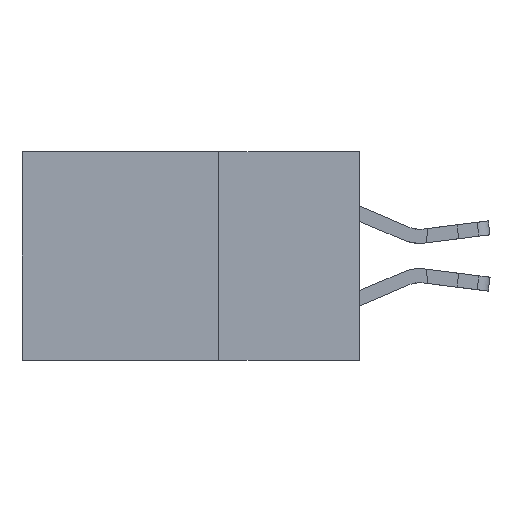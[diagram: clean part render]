
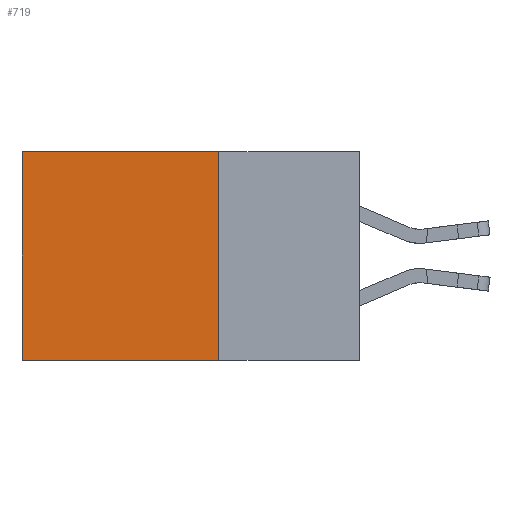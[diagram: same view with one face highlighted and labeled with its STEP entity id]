
A CAD part, left-side view. The second image highlights one B-rep face of the part: STEP entity #719.
In plain terms, the highlighted planar face has unit normal (-1, 0, 0).
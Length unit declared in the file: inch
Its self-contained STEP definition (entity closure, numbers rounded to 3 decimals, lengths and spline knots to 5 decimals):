
#719 = ADVANCED_FACE ( 'NONE', ( #21245 ), #32549, .F. ) ;
#754 = EDGE_CURVE ( 'NONE', #16952, #25200, #29790, .T. ) ;
#1808 = CARTESIAN_POINT ( 'NONE',  ( 0.2875, 0.25, 0. ) ) ;
#2608 = ORIENTED_EDGE ( 'NONE', *, *, #5707, .F. ) ;
#3145 = EDGE_CURVE ( 'NONE', #32842, #32727, #15800, .T. ) ;
#4558 = CARTESIAN_POINT ( 'NONE',  ( 0.2875, 0.6, -0.37 ) ) ;
#5681 = EDGE_LOOP ( 'NONE', ( #24630, #12362, #2608, #32507 ) ) ;
#5707 = EDGE_CURVE ( 'NONE', #16952, #32842, #6533, .T. ) ;
#6533 = LINE ( 'NONE', #10475, #29019 ) ;
#7164 = CARTESIAN_POINT ( 'NONE',  ( 0.2875, 0.25, 0. ) ) ;
#10475 = CARTESIAN_POINT ( 'NONE',  ( 0.2875, 0.25, 0. ) ) ;
#12362 = ORIENTED_EDGE ( 'NONE', *, *, #3145, .F. ) ;
#13945 = AXIS2_PLACEMENT_3D ( 'NONE', #30018, #22539, #30367 ) ;
#14082 = CARTESIAN_POINT ( 'NONE',  ( 0.2875, 0.6, 0. ) ) ;
#14201 = DIRECTION ( 'NONE',  ( 0., 0., -1. ) ) ;
#14450 = CARTESIAN_POINT ( 'NONE',  ( 0.2875, 0.25, -0.37 ) ) ;
#15681 = CARTESIAN_POINT ( 'NONE',  ( 0.2875, 0.6, 0. ) ) ;
#15800 = LINE ( 'NONE', #14450, #23179 ) ;
#15870 = CARTESIAN_POINT ( 'NONE',  ( 0.2875, 0.25, -0.37 ) ) ;
#16144 = EDGE_CURVE ( 'NONE', #25200, #32727, #16147, .T. ) ;
#16147 = LINE ( 'NONE', #14082, #29206 ) ;
#16952 = VERTEX_POINT ( 'NONE', #1808 ) ;
#21245 = FACE_OUTER_BOUND ( 'NONE', #5681, .T. ) ;
#22539 = DIRECTION ( 'NONE',  ( 1., 0., 0. ) ) ;
#22987 = DIRECTION ( 'NONE',  ( 0., 1., 0. ) ) ;
#23179 = VECTOR ( 'NONE', #30201, 39.37008 ) ;
#24630 = ORIENTED_EDGE ( 'NONE', *, *, #16144, .T. ) ;
#25200 = VERTEX_POINT ( 'NONE', #15681 ) ;
#26042 = DIRECTION ( 'NONE',  ( 0., 0., -1. ) ) ;
#29019 = VECTOR ( 'NONE', #26042, 39.37008 ) ;
#29206 = VECTOR ( 'NONE', #14201, 39.37008 ) ;
#29790 = LINE ( 'NONE', #7164, #33463 ) ;
#30018 = CARTESIAN_POINT ( 'NONE',  ( 0.2875, 0.25, 0. ) ) ;
#30201 = DIRECTION ( 'NONE',  ( 0., 1., 0. ) ) ;
#30367 = DIRECTION ( 'NONE',  ( 0., 0., -1. ) ) ;
#32507 = ORIENTED_EDGE ( 'NONE', *, *, #754, .T. ) ;
#32549 = PLANE ( 'NONE',  #13945 ) ;
#32727 = VERTEX_POINT ( 'NONE', #4558 ) ;
#32842 = VERTEX_POINT ( 'NONE', #15870 ) ;
#33463 = VECTOR ( 'NONE', #22987, 39.37008 ) ;
